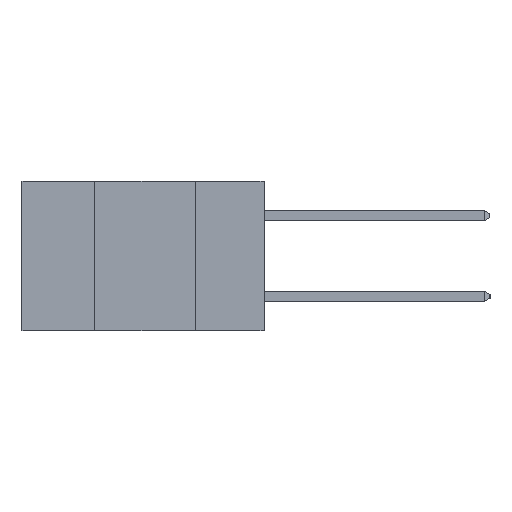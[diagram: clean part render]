
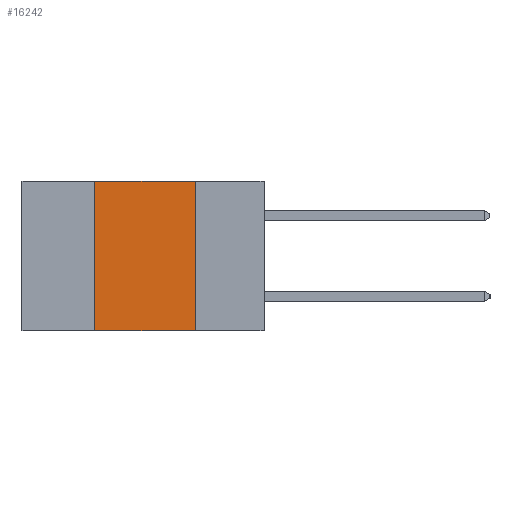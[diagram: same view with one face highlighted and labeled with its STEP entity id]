
A CAD part, left-side view. The second image highlights one B-rep face of the part: STEP entity #16242.
In plain terms, the highlighted planar face has unit normal (-1, 0, 0).
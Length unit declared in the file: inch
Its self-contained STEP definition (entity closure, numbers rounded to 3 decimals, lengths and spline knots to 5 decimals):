
#294 = VECTOR ( 'NONE', #21908, 39.37008 ) ;
#427 = ORIENTED_EDGE ( 'NONE', *, *, #14088, .T. ) ;
#2695 = DIRECTION ( 'NONE',  ( 0., -1., 0. ) ) ;
#2978 = VERTEX_POINT ( 'NONE', #7542 ) ;
#3417 = VECTOR ( 'NONE', #2695, 39.37008 ) ;
#3584 = CARTESIAN_POINT ( 'NONE',  ( 0., 0.17, -0.37 ) ) ;
#4173 = FACE_OUTER_BOUND ( 'NONE', #18429, .T. ) ;
#5067 = VERTEX_POINT ( 'NONE', #19334 ) ;
#6237 = VERTEX_POINT ( 'NONE', #8166 ) ;
#6427 = ORIENTED_EDGE ( 'NONE', *, *, #17520, .F. ) ;
#7171 = LINE ( 'NONE', #15999, #11155 ) ;
#7326 = EDGE_CURVE ( 'NONE', #5067, #2978, #13046, .T. ) ;
#7498 = LINE ( 'NONE', #14619, #3417 ) ;
#7542 = CARTESIAN_POINT ( 'NONE',  ( 0., 0.42, 0. ) ) ;
#8166 = CARTESIAN_POINT ( 'NONE',  ( 0., 0.17, 0. ) ) ;
#9270 = DIRECTION ( 'NONE',  ( 0., 0., -1. ) ) ;
#9897 = CARTESIAN_POINT ( 'NONE',  ( 0., 0.6, 0. ) ) ;
#10189 = CARTESIAN_POINT ( 'NONE',  ( 0., 0.6, 0. ) ) ;
#10751 = EDGE_CURVE ( 'NONE', #2978, #6237, #13952, .T. ) ;
#11155 = VECTOR ( 'NONE', #9270, 39.37008 ) ;
#11503 = PLANE ( 'NONE',  #20684 ) ;
#11569 = DIRECTION ( 'NONE',  ( 0., 0., -1. ) ) ;
#12012 = VECTOR ( 'NONE', #12779, 39.37008 ) ;
#12779 = DIRECTION ( 'NONE',  ( 0., 0., 1. ) ) ;
#13046 = LINE ( 'NONE', #14458, #12012 ) ;
#13952 = LINE ( 'NONE', #10189, #294 ) ;
#14088 = EDGE_CURVE ( 'NONE', #5067, #17311, #7498, .T. ) ;
#14458 = CARTESIAN_POINT ( 'NONE',  ( 0., 0.42, -0.37 ) ) ;
#14619 = CARTESIAN_POINT ( 'NONE',  ( 0., 0.6, -0.37 ) ) ;
#15999 = CARTESIAN_POINT ( 'NONE',  ( 0., 0.17, -0.37 ) ) ;
#16242 = ADVANCED_FACE ( 'NONE', ( #4173 ), #11503, .F. ) ;
#17311 = VERTEX_POINT ( 'NONE', #3584 ) ;
#17520 = EDGE_CURVE ( 'NONE', #6237, #17311, #7171, .T. ) ;
#18429 = EDGE_LOOP ( 'NONE', ( #6427, #18838, #19086, #427 ) ) ;
#18838 = ORIENTED_EDGE ( 'NONE', *, *, #10751, .F. ) ;
#19086 = ORIENTED_EDGE ( 'NONE', *, *, #7326, .F. ) ;
#19334 = CARTESIAN_POINT ( 'NONE',  ( 0., 0.42, -0.37 ) ) ;
#20684 = AXIS2_PLACEMENT_3D ( 'NONE', #9897, #21623, #11569 ) ;
#21623 = DIRECTION ( 'NONE',  ( 1., 0., 0. ) ) ;
#21908 = DIRECTION ( 'NONE',  ( 0., -1., 0. ) ) ;
